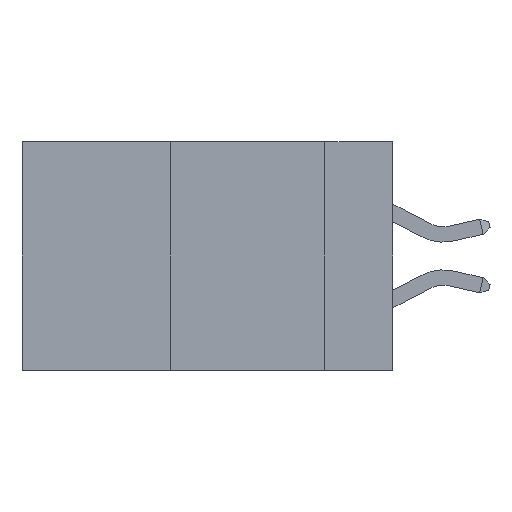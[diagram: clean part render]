
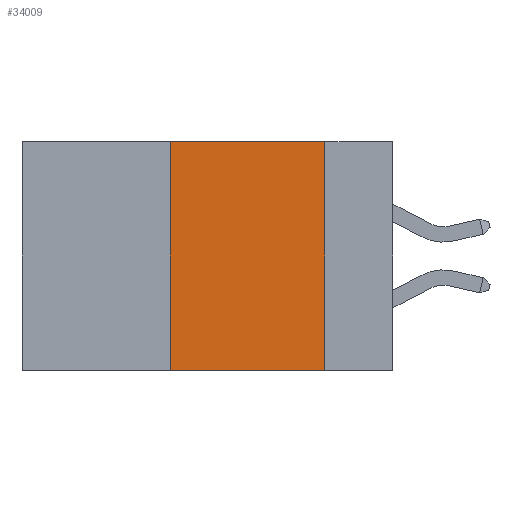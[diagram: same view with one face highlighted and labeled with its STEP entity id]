
A CAD part, left-side view. The second image highlights one B-rep face of the part: STEP entity #34009.
In plain terms, the highlighted planar face has unit normal (-1, 0, 0).
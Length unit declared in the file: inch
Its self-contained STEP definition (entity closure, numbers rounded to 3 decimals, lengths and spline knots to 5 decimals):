
#895 = LINE ( 'NONE', #25474, #7097 ) ;
#2091 = EDGE_CURVE ( 'NONE', #15182, #13313, #895, .T. ) ;
#2299 = ORIENTED_EDGE ( 'NONE', *, *, #2818, .T. ) ;
#2818 = EDGE_CURVE ( 'NONE', #32561, #12851, #7558, .T. ) ;
#3257 = CARTESIAN_POINT ( 'NONE',  ( 0., 0.11, 0. ) ) ;
#3470 = VECTOR ( 'NONE', #11557, 39.37008 ) ;
#3515 = CARTESIAN_POINT ( 'NONE',  ( 0., 0.11, 0. ) ) ;
#7097 = VECTOR ( 'NONE', #14075, 39.37008 ) ;
#7117 = CARTESIAN_POINT ( 'NONE',  ( 0., 0.6, -0.37 ) ) ;
#7558 = LINE ( 'NONE', #7117, #12576 ) ;
#7674 = CARTESIAN_POINT ( 'NONE',  ( 0., 0.36, 0. ) ) ;
#8069 = EDGE_CURVE ( 'NONE', #13313, #12851, #32300, .T. ) ;
#8322 = CARTESIAN_POINT ( 'NONE',  ( 0., 0.6, 0. ) ) ;
#10104 = VECTOR ( 'NONE', #21468, 39.37008 ) ;
#10997 = EDGE_LOOP ( 'NONE', ( #24809, #24005, #18766, #2299 ) ) ;
#11557 = DIRECTION ( 'NONE',  ( 0., 0., -1. ) ) ;
#12576 = VECTOR ( 'NONE', #17875, 39.37008 ) ;
#12851 = VERTEX_POINT ( 'NONE', #33251 ) ;
#13313 = VERTEX_POINT ( 'NONE', #3257 ) ;
#14075 = DIRECTION ( 'NONE',  ( 0., -1., 0. ) ) ;
#15182 = VERTEX_POINT ( 'NONE', #33234 ) ;
#15835 = PLANE ( 'NONE',  #28894 ) ;
#16753 = DIRECTION ( 'NONE',  ( 1., 0., 0. ) ) ;
#17875 = DIRECTION ( 'NONE',  ( 0., -1., 0. ) ) ;
#18766 = ORIENTED_EDGE ( 'NONE', *, *, #27866, .F. ) ;
#19660 = FACE_OUTER_BOUND ( 'NONE', #10997, .T. ) ;
#21468 = DIRECTION ( 'NONE',  ( 0., 0., 1. ) ) ;
#21767 = DIRECTION ( 'NONE',  ( 0., 0., -1. ) ) ;
#23964 = CARTESIAN_POINT ( 'NONE',  ( 0., 0.36, -0.37 ) ) ;
#24005 = ORIENTED_EDGE ( 'NONE', *, *, #2091, .F. ) ;
#24809 = ORIENTED_EDGE ( 'NONE', *, *, #8069, .F. ) ;
#25474 = CARTESIAN_POINT ( 'NONE',  ( 0., 0.6, 0. ) ) ;
#27866 = EDGE_CURVE ( 'NONE', #32561, #15182, #30197, .T. ) ;
#28894 = AXIS2_PLACEMENT_3D ( 'NONE', #8322, #16753, #21767 ) ;
#30197 = LINE ( 'NONE', #7674, #10104 ) ;
#32300 = LINE ( 'NONE', #3515, #3470 ) ;
#32561 = VERTEX_POINT ( 'NONE', #23964 ) ;
#33234 = CARTESIAN_POINT ( 'NONE',  ( 0., 0.36, 0. ) ) ;
#33251 = CARTESIAN_POINT ( 'NONE',  ( 0., 0.11, -0.37 ) ) ;
#34009 = ADVANCED_FACE ( 'NONE', ( #19660 ), #15835, .F. ) ;
